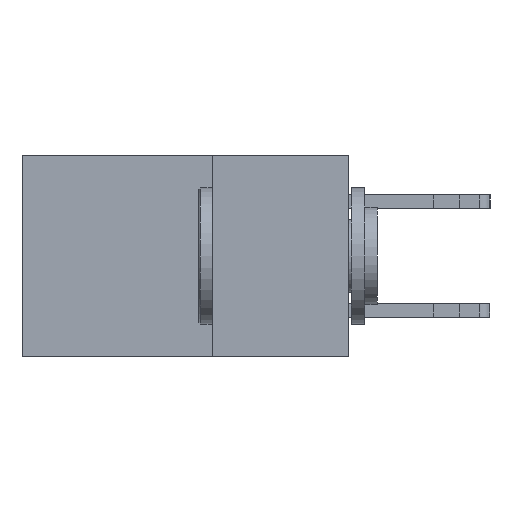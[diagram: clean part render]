
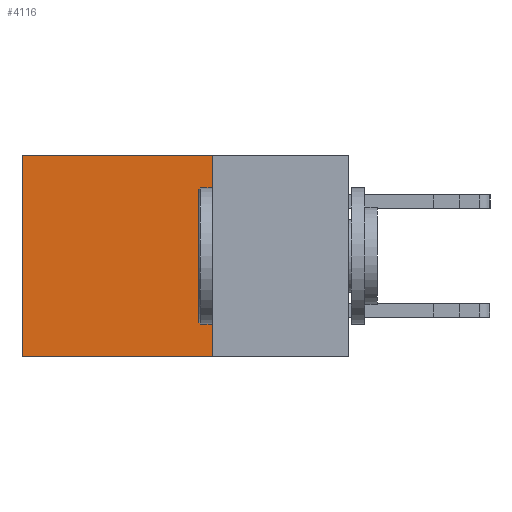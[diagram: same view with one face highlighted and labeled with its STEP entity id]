
A CAD part, left-side view. The second image highlights one B-rep face of the part: STEP entity #4116.
In plain terms, the highlighted planar face has unit normal (-1, 0, 0).
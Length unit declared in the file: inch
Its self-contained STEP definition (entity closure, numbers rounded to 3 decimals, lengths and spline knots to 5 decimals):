
#106 = DIRECTION ( 'NONE',  ( 1., 0., 0. ) ) ;
#277 = ORIENTED_EDGE ( 'NONE', *, *, #5102, .T. ) ;
#977 = EDGE_CURVE ( 'NONE', #25327, #20147, #21792, .T. ) ;
#1668 = CARTESIAN_POINT ( 'NONE',  ( 0.298, 0.25, 0. ) ) ;
#2300 = VECTOR ( 'NONE', #2772, 39.37008 ) ;
#2772 = DIRECTION ( 'NONE',  ( 0., 1., 0. ) ) ;
#3979 = VERTEX_POINT ( 'NONE', #22091 ) ;
#4116 = ADVANCED_FACE ( 'NONE', ( #12154 ), #20261, .F. ) ;
#4191 = VECTOR ( 'NONE', #22517, 39.37008 ) ;
#4345 = ORIENTED_EDGE ( 'NONE', *, *, #15530, .F. ) ;
#5102 = EDGE_CURVE ( 'NONE', #17665, #3979, #16287, .T. ) ;
#6723 = CARTESIAN_POINT ( 'NONE',  ( 0.298, 0.25, -0.37 ) ) ;
#7590 = ORIENTED_EDGE ( 'NONE', *, *, #24355, .T. ) ;
#11383 = DIRECTION ( 'NONE',  ( 0., 0., -1. ) ) ;
#11864 = CARTESIAN_POINT ( 'NONE',  ( 0.298, 0.6, 0. ) ) ;
#12154 = FACE_OUTER_BOUND ( 'NONE', #13787, .T. ) ;
#12452 = VECTOR ( 'NONE', #14916, 39.37008 ) ;
#13658 = LINE ( 'NONE', #20890, #2300 ) ;
#13787 = EDGE_LOOP ( 'NONE', ( #277, #4345, #24938, #7590 ) ) ;
#14916 = DIRECTION ( 'NONE',  ( 0., 1., 0. ) ) ;
#15530 = EDGE_CURVE ( 'NONE', #20147, #3979, #17877, .T. ) ;
#16287 = LINE ( 'NONE', #11864, #4191 ) ;
#16409 = CARTESIAN_POINT ( 'NONE',  ( 0.298, 0.25, 0. ) ) ;
#16480 = VECTOR ( 'NONE', #11383, 39.37008 ) ;
#17665 = VERTEX_POINT ( 'NONE', #18676 ) ;
#17877 = LINE ( 'NONE', #6723, #12452 ) ;
#18676 = CARTESIAN_POINT ( 'NONE',  ( 0.298, 0.6, 0. ) ) ;
#19910 = CARTESIAN_POINT ( 'NONE',  ( 0.298, 0.25, -0.37 ) ) ;
#20147 = VERTEX_POINT ( 'NONE', #19910 ) ;
#20162 = DIRECTION ( 'NONE',  ( 0., 0., -1. ) ) ;
#20254 = CARTESIAN_POINT ( 'NONE',  ( 0.298, 0.25, 0. ) ) ;
#20261 = PLANE ( 'NONE',  #24353 ) ;
#20890 = CARTESIAN_POINT ( 'NONE',  ( 0.298, 0.25, 0. ) ) ;
#21792 = LINE ( 'NONE', #1668, #16480 ) ;
#22091 = CARTESIAN_POINT ( 'NONE',  ( 0.298, 0.6, -0.37 ) ) ;
#22517 = DIRECTION ( 'NONE',  ( 0., 0., -1. ) ) ;
#24353 = AXIS2_PLACEMENT_3D ( 'NONE', #20254, #106, #20162 ) ;
#24355 = EDGE_CURVE ( 'NONE', #25327, #17665, #13658, .T. ) ;
#24938 = ORIENTED_EDGE ( 'NONE', *, *, #977, .F. ) ;
#25327 = VERTEX_POINT ( 'NONE', #16409 ) ;
